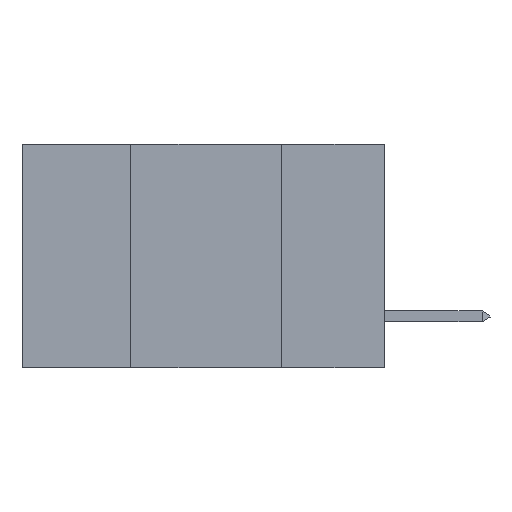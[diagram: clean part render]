
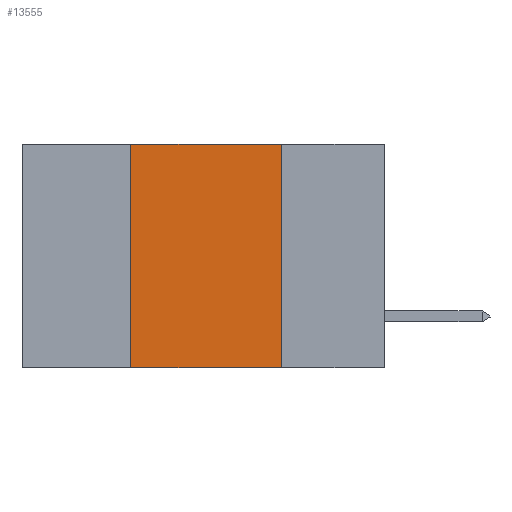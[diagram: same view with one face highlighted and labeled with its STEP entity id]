
A CAD part, left-side view. The second image highlights one B-rep face of the part: STEP entity #13555.
In plain terms, the highlighted planar face has unit normal (-1, 0, 0).
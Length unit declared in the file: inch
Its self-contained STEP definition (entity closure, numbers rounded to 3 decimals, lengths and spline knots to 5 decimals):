
#957 = VECTOR ( 'NONE', #18496, 39.37008 ) ;
#1129 = EDGE_CURVE ( 'NONE', #11439, #2129, #9296, .T. ) ;
#1947 = VERTEX_POINT ( 'NONE', #19102 ) ;
#2129 = VERTEX_POINT ( 'NONE', #12673 ) ;
#2883 = LINE ( 'NONE', #9119, #3910 ) ;
#3798 = VERTEX_POINT ( 'NONE', #7125 ) ;
#3855 = CARTESIAN_POINT ( 'NONE',  ( 0., 0.6, 0. ) ) ;
#3910 = VECTOR ( 'NONE', #15677, 39.37008 ) ;
#4076 = CARTESIAN_POINT ( 'NONE',  ( 0., 0.17, 0. ) ) ;
#5094 = AXIS2_PLACEMENT_3D ( 'NONE', #6291, #19353, #19495 ) ;
#5705 = EDGE_LOOP ( 'NONE', ( #19396, #16301, #6526, #9255 ) ) ;
#5749 = CARTESIAN_POINT ( 'NONE',  ( 0., 0.42, 0. ) ) ;
#6137 = LINE ( 'NONE', #3855, #957 ) ;
#6291 = CARTESIAN_POINT ( 'NONE',  ( 0., 0.6, 0. ) ) ;
#6526 = ORIENTED_EDGE ( 'NONE', *, *, #20296, .F. ) ;
#6808 = FACE_OUTER_BOUND ( 'NONE', #5705, .T. ) ;
#7125 = CARTESIAN_POINT ( 'NONE',  ( 0., 0.42, -0.37 ) ) ;
#9119 = CARTESIAN_POINT ( 'NONE',  ( 0., 0.6, -0.37 ) ) ;
#9255 = ORIENTED_EDGE ( 'NONE', *, *, #9538, .T. ) ;
#9296 = LINE ( 'NONE', #21085, #15209 ) ;
#9538 = EDGE_CURVE ( 'NONE', #3798, #2129, #2883, .T. ) ;
#11439 = VERTEX_POINT ( 'NONE', #4076 ) ;
#11620 = DIRECTION ( 'NONE',  ( 0., 0., -1. ) ) ;
#11821 = VECTOR ( 'NONE', #13750, 39.37008 ) ;
#12673 = CARTESIAN_POINT ( 'NONE',  ( 0., 0.17, -0.37 ) ) ;
#13555 = ADVANCED_FACE ( 'NONE', ( #6808 ), #17623, .F. ) ;
#13750 = DIRECTION ( 'NONE',  ( 0., 0., 1. ) ) ;
#15209 = VECTOR ( 'NONE', #11620, 39.37008 ) ;
#15677 = DIRECTION ( 'NONE',  ( 0., -1., 0. ) ) ;
#16301 = ORIENTED_EDGE ( 'NONE', *, *, #18625, .F. ) ;
#17623 = PLANE ( 'NONE',  #5094 ) ;
#18496 = DIRECTION ( 'NONE',  ( 0., -1., 0. ) ) ;
#18625 = EDGE_CURVE ( 'NONE', #1947, #11439, #6137, .T. ) ;
#19102 = CARTESIAN_POINT ( 'NONE',  ( 0., 0.42, 0. ) ) ;
#19353 = DIRECTION ( 'NONE',  ( 1., 0., 0. ) ) ;
#19396 = ORIENTED_EDGE ( 'NONE', *, *, #1129, .F. ) ;
#19495 = DIRECTION ( 'NONE',  ( 0., 0., -1. ) ) ;
#20296 = EDGE_CURVE ( 'NONE', #3798, #1947, #20688, .T. ) ;
#20688 = LINE ( 'NONE', #5749, #11821 ) ;
#21085 = CARTESIAN_POINT ( 'NONE',  ( 0., 0.17, 0. ) ) ;
